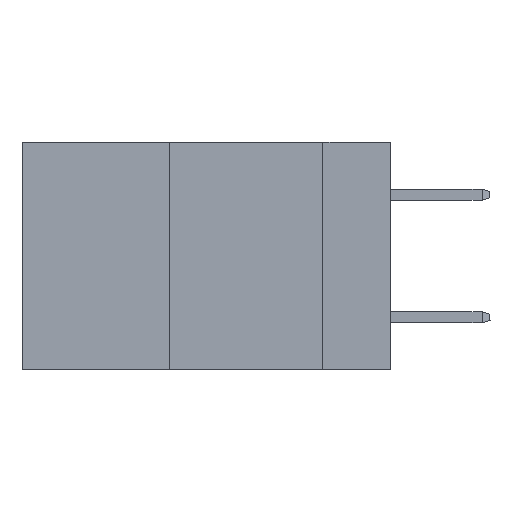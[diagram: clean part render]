
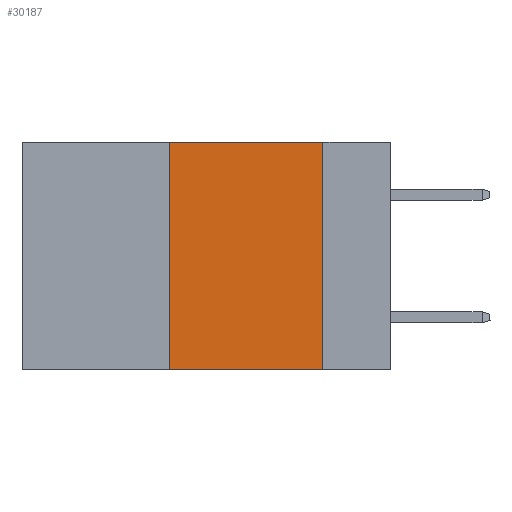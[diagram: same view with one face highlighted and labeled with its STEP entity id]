
A CAD part, left-side view. The second image highlights one B-rep face of the part: STEP entity #30187.
In plain terms, the highlighted planar face has unit normal (-1, 0, 0).
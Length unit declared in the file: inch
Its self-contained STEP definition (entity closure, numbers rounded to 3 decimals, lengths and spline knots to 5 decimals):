
#1346 = CARTESIAN_POINT ( 'NONE',  ( 0., 0.6, 0. ) ) ;
#1878 = CARTESIAN_POINT ( 'NONE',  ( 0., 0.6, -0.37 ) ) ;
#2374 = DIRECTION ( 'NONE',  ( 0., -1., 0. ) ) ;
#3324 = ORIENTED_EDGE ( 'NONE', *, *, #10742, .F. ) ;
#3991 = VERTEX_POINT ( 'NONE', #20804 ) ;
#4631 = FACE_OUTER_BOUND ( 'NONE', #6514, .T. ) ;
#5771 = DIRECTION ( 'NONE',  ( 0., 0., -1. ) ) ;
#6514 = EDGE_LOOP ( 'NONE', ( #28474, #23529, #3324, #17313 ) ) ;
#7285 = DIRECTION ( 'NONE',  ( 0., 0., -1. ) ) ;
#7984 = VECTOR ( 'NONE', #11632, 39.37008 ) ;
#8145 = LINE ( 'NONE', #16888, #32714 ) ;
#9966 = VERTEX_POINT ( 'NONE', #35628 ) ;
#10742 = EDGE_CURVE ( 'NONE', #9966, #3991, #8145, .T. ) ;
#11627 = LINE ( 'NONE', #11992, #7984 ) ;
#11632 = DIRECTION ( 'NONE',  ( 0., -1., 0. ) ) ;
#11992 = CARTESIAN_POINT ( 'NONE',  ( 0., 0.6, 0. ) ) ;
#13135 = DIRECTION ( 'NONE',  ( 1., 0., 0. ) ) ;
#16525 = VERTEX_POINT ( 'NONE', #36299 ) ;
#16813 = EDGE_CURVE ( 'NONE', #3991, #16525, #11627, .T. ) ;
#16888 = CARTESIAN_POINT ( 'NONE',  ( 0., 0.36, 0. ) ) ;
#17313 = ORIENTED_EDGE ( 'NONE', *, *, #30242, .T. ) ;
#18087 = VECTOR ( 'NONE', #5771, 39.37008 ) ;
#18484 = CARTESIAN_POINT ( 'NONE',  ( 0., 0.11, -0.37 ) ) ;
#18520 = EDGE_CURVE ( 'NONE', #16525, #30021, #20817, .T. ) ;
#20804 = CARTESIAN_POINT ( 'NONE',  ( 0., 0.36, 0. ) ) ;
#20817 = LINE ( 'NONE', #29172, #18087 ) ;
#22996 = DIRECTION ( 'NONE',  ( 0., 0., 1. ) ) ;
#23529 = ORIENTED_EDGE ( 'NONE', *, *, #16813, .F. ) ;
#25092 = PLANE ( 'NONE',  #37640 ) ;
#27877 = VECTOR ( 'NONE', #2374, 39.37008 ) ;
#28474 = ORIENTED_EDGE ( 'NONE', *, *, #18520, .F. ) ;
#29172 = CARTESIAN_POINT ( 'NONE',  ( 0., 0.11, 0. ) ) ;
#30021 = VERTEX_POINT ( 'NONE', #18484 ) ;
#30187 = ADVANCED_FACE ( 'NONE', ( #4631 ), #25092, .F. ) ;
#30242 = EDGE_CURVE ( 'NONE', #9966, #30021, #35581, .T. ) ;
#32714 = VECTOR ( 'NONE', #22996, 39.37008 ) ;
#35581 = LINE ( 'NONE', #1878, #27877 ) ;
#35628 = CARTESIAN_POINT ( 'NONE',  ( 0., 0.36, -0.37 ) ) ;
#36299 = CARTESIAN_POINT ( 'NONE',  ( 0., 0.11, 0. ) ) ;
#37640 = AXIS2_PLACEMENT_3D ( 'NONE', #1346, #13135, #7285 ) ;
